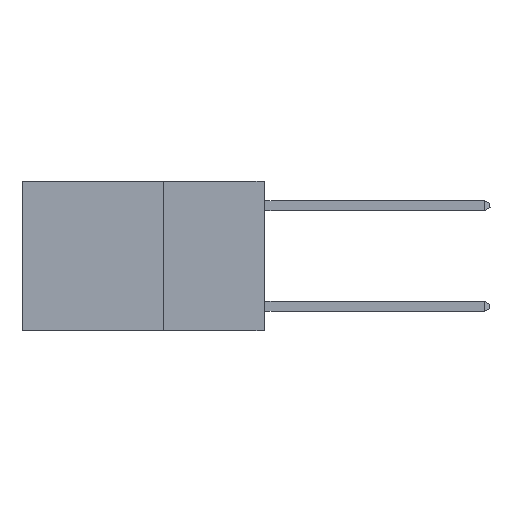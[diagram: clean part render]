
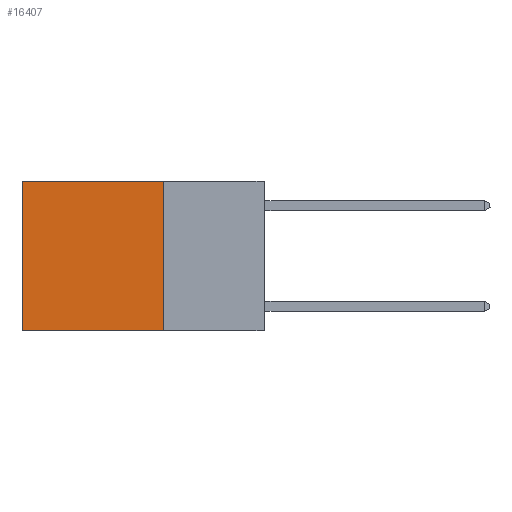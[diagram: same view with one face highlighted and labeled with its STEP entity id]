
A CAD part, left-side view. The second image highlights one B-rep face of the part: STEP entity #16407.
In plain terms, the highlighted planar face has unit normal (-1, 0, 0).
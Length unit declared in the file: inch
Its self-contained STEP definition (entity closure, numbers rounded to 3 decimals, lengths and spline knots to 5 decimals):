
#498 = CARTESIAN_POINT ( 'NONE',  ( 0.2625, 0.25, 0. ) ) ;
#1152 = VECTOR ( 'NONE', #5917, 39.37008 ) ;
#1552 = CARTESIAN_POINT ( 'NONE',  ( 0.2625, 0.25, 0. ) ) ;
#1856 = VERTEX_POINT ( 'NONE', #4456 ) ;
#2983 = EDGE_CURVE ( 'NONE', #3938, #3050, #9129, .T. ) ;
#3050 = VERTEX_POINT ( 'NONE', #10517 ) ;
#3111 = VECTOR ( 'NONE', #16305, 39.37008 ) ;
#3438 = PLANE ( 'NONE',  #15650 ) ;
#3814 = EDGE_CURVE ( 'NONE', #3050, #1856, #10367, .T. ) ;
#3938 = VERTEX_POINT ( 'NONE', #1552 ) ;
#4335 = CARTESIAN_POINT ( 'NONE',  ( 0.2625, 0.6, 0. ) ) ;
#4456 = CARTESIAN_POINT ( 'NONE',  ( 0.2625, 0.6, -0.37 ) ) ;
#4785 = LINE ( 'NONE', #498, #1152 ) ;
#5286 = EDGE_LOOP ( 'NONE', ( #15418, #15526, #15932, #9171 ) ) ;
#5917 = DIRECTION ( 'NONE',  ( 0., 0., -1. ) ) ;
#6048 = CARTESIAN_POINT ( 'NONE',  ( 0.2625, 0.25, -0.37 ) ) ;
#6108 = DIRECTION ( 'NONE',  ( 1., 0., 0. ) ) ;
#6936 = VECTOR ( 'NONE', #12115, 39.37008 ) ;
#7550 = EDGE_CURVE ( 'NONE', #3938, #16398, #4785, .T. ) ;
#8438 = CARTESIAN_POINT ( 'NONE',  ( 0.2625, 0.25, -0.37 ) ) ;
#8731 = VECTOR ( 'NONE', #13065, 39.37008 ) ;
#9129 = LINE ( 'NONE', #16946, #8731 ) ;
#9171 = ORIENTED_EDGE ( 'NONE', *, *, #2983, .T. ) ;
#10367 = LINE ( 'NONE', #4335, #6936 ) ;
#10517 = CARTESIAN_POINT ( 'NONE',  ( 0.2625, 0.6, 0. ) ) ;
#12115 = DIRECTION ( 'NONE',  ( 0., 0., -1. ) ) ;
#13065 = DIRECTION ( 'NONE',  ( 0., 1., 0. ) ) ;
#13182 = FACE_OUTER_BOUND ( 'NONE', #5286, .T. ) ;
#13904 = CARTESIAN_POINT ( 'NONE',  ( 0.2625, 0.25, 0. ) ) ;
#13917 = EDGE_CURVE ( 'NONE', #16398, #1856, #16633, .T. ) ;
#15234 = DIRECTION ( 'NONE',  ( 0., 0., -1. ) ) ;
#15418 = ORIENTED_EDGE ( 'NONE', *, *, #3814, .T. ) ;
#15526 = ORIENTED_EDGE ( 'NONE', *, *, #13917, .F. ) ;
#15650 = AXIS2_PLACEMENT_3D ( 'NONE', #13904, #6108, #15234 ) ;
#15932 = ORIENTED_EDGE ( 'NONE', *, *, #7550, .F. ) ;
#16305 = DIRECTION ( 'NONE',  ( 0., 1., 0. ) ) ;
#16398 = VERTEX_POINT ( 'NONE', #6048 ) ;
#16407 = ADVANCED_FACE ( 'NONE', ( #13182 ), #3438, .F. ) ;
#16633 = LINE ( 'NONE', #8438, #3111 ) ;
#16946 = CARTESIAN_POINT ( 'NONE',  ( 0.2625, 0.25, 0. ) ) ;
